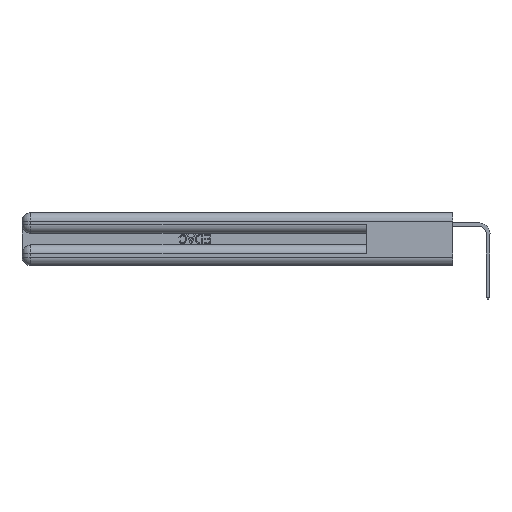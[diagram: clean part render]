
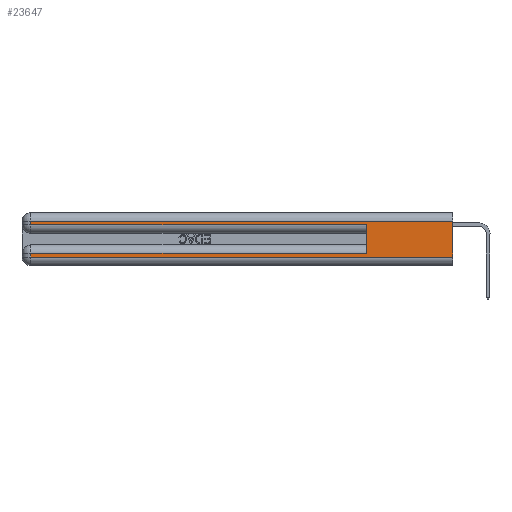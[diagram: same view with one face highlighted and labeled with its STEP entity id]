
A CAD part, left-side view. The second image highlights one B-rep face of the part: STEP entity #23647.
In plain terms, the highlighted planar face has unit normal (-1, 0, 0).
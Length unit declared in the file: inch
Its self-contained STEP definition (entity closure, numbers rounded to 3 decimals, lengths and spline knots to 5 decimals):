
#460 = DIRECTION ( 'NONE',  ( 1., 0., 0. ) ) ;
#1586 = EDGE_CURVE ( 'NONE', #33649, #21367, #29909, .T. ) ;
#2076 = EDGE_CURVE ( 'NONE', #21367, #19162, #3198, .T. ) ;
#2092 = EDGE_CURVE ( 'NONE', #33902, #29347, #34053, .T. ) ;
#2262 = CARTESIAN_POINT ( 'NONE',  ( 0., 2.94, 0.31 ) ) ;
#2279 = VECTOR ( 'NONE', #2682, 39.37008 ) ;
#2552 = FACE_OUTER_BOUND ( 'NONE', #4587, .T. ) ;
#2682 = DIRECTION ( 'NONE',  ( 0., 1., 0. ) ) ;
#3198 = LINE ( 'NONE', #5561, #26196 ) ;
#4587 = EDGE_LOOP ( 'NONE', ( #28340, #14795, #14181, #23662, #34425, #29249, #27790, #13323 ) ) ;
#4774 = CARTESIAN_POINT ( 'NONE',  ( 0., 0.6, 0.085 ) ) ;
#4961 = DIRECTION ( 'NONE',  ( 0., 0., 1. ) ) ;
#5098 = DIRECTION ( 'NONE',  ( 0., 0., -1. ) ) ;
#5561 = CARTESIAN_POINT ( 'NONE',  ( 0., 2.94, 0.37 ) ) ;
#6430 = CARTESIAN_POINT ( 'NONE',  ( 0., 0., 0.37 ) ) ;
#11859 = AXIS2_PLACEMENT_3D ( 'NONE', #6430, #460, #21529 ) ;
#13323 = ORIENTED_EDGE ( 'NONE', *, *, #15956, .T. ) ;
#14181 = ORIENTED_EDGE ( 'NONE', *, *, #29170, .T. ) ;
#14286 = VECTOR ( 'NONE', #14298, 39.37008 ) ;
#14298 = DIRECTION ( 'NONE',  ( 0., -1., 0. ) ) ;
#14467 = CARTESIAN_POINT ( 'NONE',  ( 0., 0.6, 0.285 ) ) ;
#14795 = ORIENTED_EDGE ( 'NONE', *, *, #2092, .T. ) ;
#14799 = CARTESIAN_POINT ( 'NONE',  ( 0., 0., 0.06 ) ) ;
#15420 = LINE ( 'NONE', #20231, #22514 ) ;
#15942 = LINE ( 'NONE', #28071, #25820 ) ;
#15956 = EDGE_CURVE ( 'NONE', #19162, #29185, #16329, .T. ) ;
#16215 = VERTEX_POINT ( 'NONE', #19045 ) ;
#16329 = LINE ( 'NONE', #14799, #25266 ) ;
#19045 = CARTESIAN_POINT ( 'NONE',  ( 0., 2.94, 0.285 ) ) ;
#19162 = VERTEX_POINT ( 'NONE', #32937 ) ;
#20231 = CARTESIAN_POINT ( 'NONE',  ( 0., 0., 0.37 ) ) ;
#21367 = VERTEX_POINT ( 'NONE', #26274 ) ;
#21529 = DIRECTION ( 'NONE',  ( 0., 0., -1. ) ) ;
#21959 = DIRECTION ( 'NONE',  ( 0., 0., -1. ) ) ;
#22514 = VECTOR ( 'NONE', #5098, 39.37008 ) ;
#23647 = ADVANCED_FACE ( 'NONE', ( #2552 ), #36308, .F. ) ;
#23662 = ORIENTED_EDGE ( 'NONE', *, *, #38101, .T. ) ;
#23984 = EDGE_CURVE ( 'NONE', #33649, #36552, #29234, .T. ) ;
#24245 = DIRECTION ( 'NONE',  ( 0., 1., 0. ) ) ;
#25266 = VECTOR ( 'NONE', #38639, 39.37008 ) ;
#25820 = VECTOR ( 'NONE', #21959, 39.37008 ) ;
#26196 = VECTOR ( 'NONE', #29534, 39.37008 ) ;
#26274 = CARTESIAN_POINT ( 'NONE',  ( 0., 2.94, 0.085 ) ) ;
#26389 = CARTESIAN_POINT ( 'NONE',  ( 0., 0., 0.285 ) ) ;
#27790 = ORIENTED_EDGE ( 'NONE', *, *, #2076, .T. ) ;
#28071 = CARTESIAN_POINT ( 'NONE',  ( 0., 2.94, 0.37 ) ) ;
#28340 = ORIENTED_EDGE ( 'NONE', *, *, #35940, .F. ) ;
#29170 = EDGE_CURVE ( 'NONE', #29347, #16215, #15942, .T. ) ;
#29185 = VERTEX_POINT ( 'NONE', #31193 ) ;
#29234 = LINE ( 'NONE', #34849, #37095 ) ;
#29249 = ORIENTED_EDGE ( 'NONE', *, *, #1586, .T. ) ;
#29347 = VERTEX_POINT ( 'NONE', #2262 ) ;
#29534 = DIRECTION ( 'NONE',  ( 0., 0., -1. ) ) ;
#29909 = LINE ( 'NONE', #36002, #36844 ) ;
#31193 = CARTESIAN_POINT ( 'NONE',  ( 0., 0., 0.06 ) ) ;
#32503 = CARTESIAN_POINT ( 'NONE',  ( 0., 0., 0.31 ) ) ;
#32854 = CARTESIAN_POINT ( 'NONE',  ( 0., 0., 0.31 ) ) ;
#32937 = CARTESIAN_POINT ( 'NONE',  ( 0., 2.94, 0.06 ) ) ;
#33649 = VERTEX_POINT ( 'NONE', #4774 ) ;
#33902 = VERTEX_POINT ( 'NONE', #32854 ) ;
#34053 = LINE ( 'NONE', #32503, #2279 ) ;
#34425 = ORIENTED_EDGE ( 'NONE', *, *, #23984, .F. ) ;
#34849 = CARTESIAN_POINT ( 'NONE',  ( 0., 0.6, 0.145 ) ) ;
#35940 = EDGE_CURVE ( 'NONE', #33902, #29185, #15420, .T. ) ;
#36002 = CARTESIAN_POINT ( 'NONE',  ( 0., 0., 0.085 ) ) ;
#36308 = PLANE ( 'NONE',  #11859 ) ;
#36552 = VERTEX_POINT ( 'NONE', #14467 ) ;
#36844 = VECTOR ( 'NONE', #24245, 39.37008 ) ;
#37095 = VECTOR ( 'NONE', #4961, 39.37008 ) ;
#38076 = LINE ( 'NONE', #26389, #14286 ) ;
#38101 = EDGE_CURVE ( 'NONE', #16215, #36552, #38076, .T. ) ;
#38639 = DIRECTION ( 'NONE',  ( 0., -1., 0. ) ) ;
